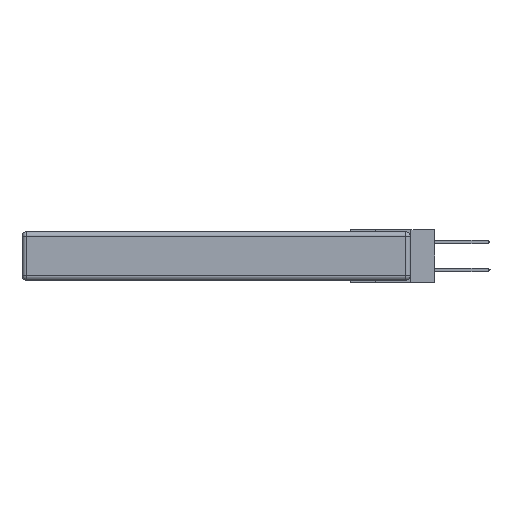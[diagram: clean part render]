
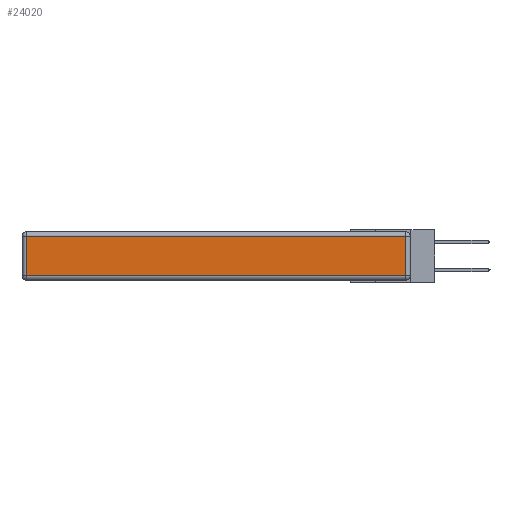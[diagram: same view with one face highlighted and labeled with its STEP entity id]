
A CAD part, left-side view. The second image highlights one B-rep face of the part: STEP entity #24020.
In plain terms, the highlighted planar face has unit normal (-1, 0, 0).
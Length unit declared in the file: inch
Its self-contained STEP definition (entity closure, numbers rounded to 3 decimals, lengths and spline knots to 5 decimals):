
#1132 = VECTOR ( 'NONE', #8642, 39.37008 ) ;
#2637 = CARTESIAN_POINT ( 'NONE',  ( 0., 0.03, -0.343 ) ) ;
#2851 = ORIENTED_EDGE ( 'NONE', *, *, #18203, .T. ) ;
#4688 = CARTESIAN_POINT ( 'NONE',  ( 0., 0., -0.313 ) ) ;
#4706 = VERTEX_POINT ( 'NONE', #24554 ) ;
#6400 = ORIENTED_EDGE ( 'NONE', *, *, #16464, .T. ) ;
#6644 = DIRECTION ( 'NONE',  ( 0., 0., 1. ) ) ;
#7188 = CARTESIAN_POINT ( 'NONE',  ( 0., 2.75, -0.03 ) ) ;
#7337 = VERTEX_POINT ( 'NONE', #21778 ) ;
#7621 = EDGE_CURVE ( 'NONE', #16696, #8893, #12663, .T. ) ;
#8440 = CARTESIAN_POINT ( 'NONE',  ( 0., 2.72, -0.343 ) ) ;
#8642 = DIRECTION ( 'NONE',  ( 0., 0., 1. ) ) ;
#8893 = VERTEX_POINT ( 'NONE', #26675 ) ;
#9862 = VECTOR ( 'NONE', #15225, 39.37008 ) ;
#10484 = FACE_OUTER_BOUND ( 'NONE', #21447, .T. ) ;
#10972 = AXIS2_PLACEMENT_3D ( 'NONE', #13035, #11134, #6644 ) ;
#11134 = DIRECTION ( 'NONE',  ( -1., 0., 0. ) ) ;
#11920 = CARTESIAN_POINT ( 'NONE',  ( 0., 0.03, -0.313 ) ) ;
#12487 = LINE ( 'NONE', #8440, #13781 ) ;
#12575 = EDGE_CURVE ( 'NONE', #7337, #16696, #19213, .T. ) ;
#12663 = LINE ( 'NONE', #2637, #1132 ) ;
#13035 = CARTESIAN_POINT ( 'NONE',  ( 0., 0., -0.343 ) ) ;
#13607 = ORIENTED_EDGE ( 'NONE', *, *, #7621, .T. ) ;
#13781 = VECTOR ( 'NONE', #23020, 39.37008 ) ;
#15225 = DIRECTION ( 'NONE',  ( 0., 1., 0. ) ) ;
#16464 = EDGE_CURVE ( 'NONE', #4706, #7337, #12487, .T. ) ;
#16696 = VERTEX_POINT ( 'NONE', #11920 ) ;
#18203 = EDGE_CURVE ( 'NONE', #8893, #4706, #26118, .T. ) ;
#19213 = LINE ( 'NONE', #4688, #25713 ) ;
#19344 = ORIENTED_EDGE ( 'NONE', *, *, #12575, .T. ) ;
#19346 = PLANE ( 'NONE',  #10972 ) ;
#21447 = EDGE_LOOP ( 'NONE', ( #19344, #13607, #2851, #6400 ) ) ;
#21778 = CARTESIAN_POINT ( 'NONE',  ( 0., 2.72, -0.313 ) ) ;
#23020 = DIRECTION ( 'NONE',  ( 0., 0., -1. ) ) ;
#24020 = ADVANCED_FACE ( 'NONE', ( #10484 ), #19346, .T. ) ;
#24554 = CARTESIAN_POINT ( 'NONE',  ( 0., 2.72, -0.03 ) ) ;
#25713 = VECTOR ( 'NONE', #25772, 39.37008 ) ;
#25772 = DIRECTION ( 'NONE',  ( 0., -1., 0. ) ) ;
#26118 = LINE ( 'NONE', #7188, #9862 ) ;
#26675 = CARTESIAN_POINT ( 'NONE',  ( 0., 0.03, -0.03 ) ) ;
